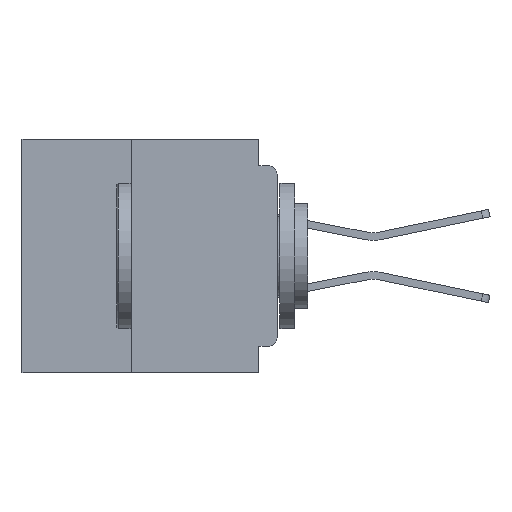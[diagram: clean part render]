
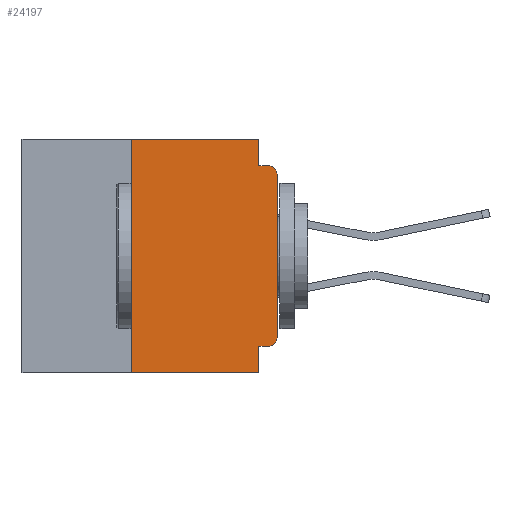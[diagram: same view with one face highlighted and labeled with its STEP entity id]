
A CAD part, left-side view. The second image highlights one B-rep face of the part: STEP entity #24197.
In plain terms, the highlighted planar face has unit normal (-1, 0, 0).
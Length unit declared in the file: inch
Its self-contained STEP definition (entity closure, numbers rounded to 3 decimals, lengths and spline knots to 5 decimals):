
#106 = DIRECTION ( 'NONE',  ( 0., 0., -1. ) ) ;
#341 = EDGE_CURVE ( 'NONE', #32943, #8688, #2391, .T. ) ;
#400 = CARTESIAN_POINT ( 'NONE',  ( 0., 0.031, -0.045 ) ) ;
#978 = EDGE_CURVE ( 'NONE', #24686, #35178, #29564, .T. ) ;
#1433 = ORIENTED_EDGE ( 'NONE', *, *, #11013, .T. ) ;
#2391 = LINE ( 'NONE', #38755, #8771 ) ;
#2844 = CARTESIAN_POINT ( 'NONE',  ( 0., 0.031, -0.355 ) ) ;
#2894 = CARTESIAN_POINT ( 'NONE',  ( 0., 0.031, 0. ) ) ;
#3138 = CARTESIAN_POINT ( 'NONE',  ( 0., 0.25, -0.4 ) ) ;
#3370 = LINE ( 'NONE', #31686, #35425 ) ;
#4329 = VECTOR ( 'NONE', #9889, 39.37008 ) ;
#4884 = ORIENTED_EDGE ( 'NONE', *, *, #978, .F. ) ;
#4957 = VECTOR ( 'NONE', #106, 39.37008 ) ;
#6309 = CARTESIAN_POINT ( 'NONE',  ( 0., 0., -0.355 ) ) ;
#6928 = EDGE_LOOP ( 'NONE', ( #15433, #33635, #37844, #12957, #4884, #15683, #9833, #31314, #25213, #1433 ) ) ;
#8688 = VERTEX_POINT ( 'NONE', #25031 ) ;
#8771 = VECTOR ( 'NONE', #22029, 39.37008 ) ;
#9060 = CARTESIAN_POINT ( 'NONE',  ( 0., 0.015, -0.34 ) ) ;
#9833 = ORIENTED_EDGE ( 'NONE', *, *, #341, .T. ) ;
#9889 = DIRECTION ( 'NONE',  ( 0., 0., 1. ) ) ;
#11013 = EDGE_CURVE ( 'NONE', #36621, #30843, #38886, .T. ) ;
#12176 = DIRECTION ( 'NONE',  ( 0., 0., -1. ) ) ;
#12957 = ORIENTED_EDGE ( 'NONE', *, *, #26987, .F. ) ;
#14900 = EDGE_CURVE ( 'NONE', #33015, #21269, #25139, .T. ) ;
#15433 = ORIENTED_EDGE ( 'NONE', *, *, #38281, .T. ) ;
#15683 = ORIENTED_EDGE ( 'NONE', *, *, #17863, .F. ) ;
#15999 = CARTESIAN_POINT ( 'NONE',  ( 0., 0., -0.34 ) ) ;
#16046 = CARTESIAN_POINT ( 'NONE',  ( 0., 0., 0. ) ) ;
#16359 = CARTESIAN_POINT ( 'NONE',  ( 0., 0.015, -0.355 ) ) ;
#16915 = VERTEX_POINT ( 'NONE', #39492 ) ;
#17385 = DIRECTION ( 'NONE',  ( -1., 0., 0. ) ) ;
#17863 = EDGE_CURVE ( 'NONE', #32943, #24686, #25382, .T. ) ;
#18471 = LINE ( 'NONE', #6309, #33891 ) ;
#18742 = CARTESIAN_POINT ( 'NONE',  ( 0., 0.015, -0.045 ) ) ;
#20249 = CARTESIAN_POINT ( 'NONE',  ( 0., 0.25, 0. ) ) ;
#20965 = DIRECTION ( 'NONE',  ( 1., 0., 0. ) ) ;
#21021 = LINE ( 'NONE', #16046, #4329 ) ;
#21269 = VERTEX_POINT ( 'NONE', #18742 ) ;
#21417 = FACE_OUTER_BOUND ( 'NONE', #6928, .T. ) ;
#22029 = DIRECTION ( 'NONE',  ( 0., -1., 0. ) ) ;
#22036 = CARTESIAN_POINT ( 'NONE',  ( 0., 0.031, 0. ) ) ;
#23772 = EDGE_CURVE ( 'NONE', #36621, #28870, #18471, .T. ) ;
#24197 = ADVANCED_FACE ( 'NONE', ( #21417 ), #30157, .F. ) ;
#24686 = VERTEX_POINT ( 'NONE', #20249 ) ;
#25031 = CARTESIAN_POINT ( 'NONE',  ( 0., 0.031, -0.4 ) ) ;
#25139 = LINE ( 'NONE', #29682, #32301 ) ;
#25213 = ORIENTED_EDGE ( 'NONE', *, *, #23772, .F. ) ;
#25382 = LINE ( 'NONE', #30788, #31570 ) ;
#26706 = VECTOR ( 'NONE', #38126, 39.37008 ) ;
#26987 = EDGE_CURVE ( 'NONE', #35178, #33015, #28779, .T. ) ;
#27093 = CARTESIAN_POINT ( 'NONE',  ( 0., 0.437, 0. ) ) ;
#28766 = AXIS2_PLACEMENT_3D ( 'NONE', #27093, #20965, #33271 ) ;
#28779 = LINE ( 'NONE', #22036, #4957 ) ;
#28870 = VERTEX_POINT ( 'NONE', #2844 ) ;
#29564 = LINE ( 'NONE', #38808, #26706 ) ;
#29682 = CARTESIAN_POINT ( 'NONE',  ( 0., 0., -0.045 ) ) ;
#29709 = AXIS2_PLACEMENT_3D ( 'NONE', #9060, #30704, #12176 ) ;
#30157 = PLANE ( 'NONE',  #28766 ) ;
#30704 = DIRECTION ( 'NONE',  ( -1., 0., 0. ) ) ;
#30788 = CARTESIAN_POINT ( 'NONE',  ( 0., 0.25, -0.4 ) ) ;
#30843 = VERTEX_POINT ( 'NONE', #15999 ) ;
#31114 = DIRECTION ( 'NONE',  ( 0., 1., 0. ) ) ;
#31314 = ORIENTED_EDGE ( 'NONE', *, *, #37830, .F. ) ;
#31570 = VECTOR ( 'NONE', #36969, 39.37008 ) ;
#31686 = CARTESIAN_POINT ( 'NONE',  ( 0., 0.031, -0.4 ) ) ;
#32301 = VECTOR ( 'NONE', #32790, 39.37008 ) ;
#32790 = DIRECTION ( 'NONE',  ( 0., -1., 0. ) ) ;
#32943 = VERTEX_POINT ( 'NONE', #3138 ) ;
#33015 = VERTEX_POINT ( 'NONE', #400 ) ;
#33066 = AXIS2_PLACEMENT_3D ( 'NONE', #35831, #17385, #38907 ) ;
#33271 = DIRECTION ( 'NONE',  ( 0., 0., -1. ) ) ;
#33531 = CIRCLE ( 'NONE', #33066, 0.015 ) ;
#33635 = ORIENTED_EDGE ( 'NONE', *, *, #37432, .T. ) ;
#33891 = VECTOR ( 'NONE', #31114, 39.37008 ) ;
#35178 = VERTEX_POINT ( 'NONE', #2894 ) ;
#35425 = VECTOR ( 'NONE', #37866, 39.37008 ) ;
#35831 = CARTESIAN_POINT ( 'NONE',  ( 0., 0.015, -0.06 ) ) ;
#36621 = VERTEX_POINT ( 'NONE', #16359 ) ;
#36969 = DIRECTION ( 'NONE',  ( 0., 0., 1. ) ) ;
#37432 = EDGE_CURVE ( 'NONE', #16915, #21269, #33531, .T. ) ;
#37830 = EDGE_CURVE ( 'NONE', #28870, #8688, #3370, .T. ) ;
#37844 = ORIENTED_EDGE ( 'NONE', *, *, #14900, .F. ) ;
#37866 = DIRECTION ( 'NONE',  ( 0., 0., -1. ) ) ;
#38126 = DIRECTION ( 'NONE',  ( 0., -1., 0. ) ) ;
#38281 = EDGE_CURVE ( 'NONE', #30843, #16915, #21021, .T. ) ;
#38755 = CARTESIAN_POINT ( 'NONE',  ( 0., 0.437, -0.4 ) ) ;
#38808 = CARTESIAN_POINT ( 'NONE',  ( 0., 0.437, 0. ) ) ;
#38886 = CIRCLE ( 'NONE', #29709, 0.015 ) ;
#38907 = DIRECTION ( 'NONE',  ( 0., 0., -1. ) ) ;
#39492 = CARTESIAN_POINT ( 'NONE',  ( 0., 0., -0.06 ) ) ;
